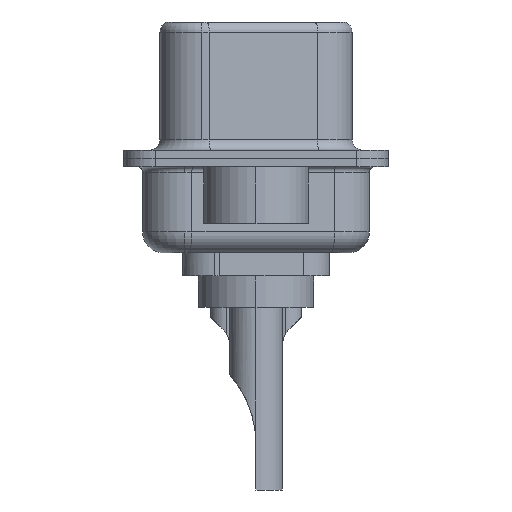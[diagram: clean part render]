
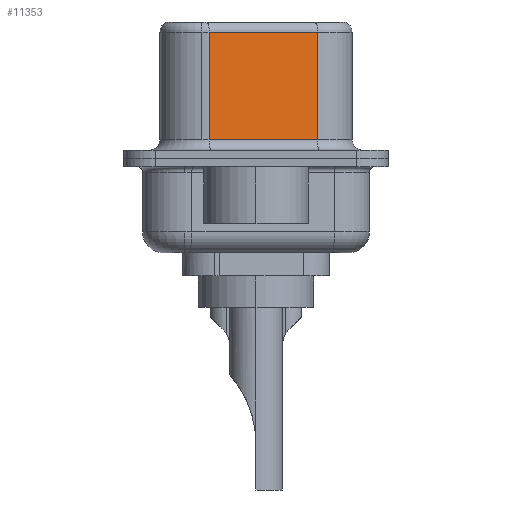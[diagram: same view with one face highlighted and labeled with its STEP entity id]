
A CAD part, left-side view. The second image highlights one B-rep face of the part: STEP entity #11353.
In plain terms, the highlighted planar face has unit normal (-0.985, -0.174, 0).
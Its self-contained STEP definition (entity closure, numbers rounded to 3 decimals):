
#414 = VERTEX_POINT ( 'NONE', #11921 ) ;
#579 = VERTEX_POINT ( 'NONE', #12509 ) ;
#940 = LINE ( 'NONE', #13242, #16454 ) ;
#2225 = ORIENTED_EDGE ( 'NONE', *, *, #14039, .T. ) ;
#2245 = CARTESIAN_POINT ( 'NONE',  ( 4.585, -2.927, 6.02 ) ) ;
#2820 = DIRECTION ( 'NONE',  ( 0., 0., -1. ) ) ;
#2828 = LINE ( 'NONE', #16336, #4476 ) ;
#3427 = EDGE_CURVE ( 'NONE', #15563, #5354, #940, .T. ) ;
#3500 = PLANE ( 'NONE',  #6195 ) ;
#3525 = CARTESIAN_POINT ( 'NONE',  ( 3.675, 2.233, 6.52 ) ) ;
#4476 = VECTOR ( 'NONE', #2820, 1000. ) ;
#4582 = EDGE_LOOP ( 'NONE', ( #11446, #7759, #16060, #2225 ) ) ;
#4767 = EDGE_CURVE ( 'NONE', #15563, #414, #2828, .T. ) ;
#5354 = VERTEX_POINT ( 'NONE', #12148 ) ;
#5702 = LINE ( 'NONE', #19414, #15691 ) ;
#6195 = AXIS2_PLACEMENT_3D ( 'NONE', #6426, #10901, #18558 ) ;
#6426 = CARTESIAN_POINT ( 'NONE',  ( 4.585, -2.927, 6.52 ) ) ;
#7759 = ORIENTED_EDGE ( 'NONE', *, *, #3427, .T. ) ;
#8699 = VECTOR ( 'NONE', #12587, 1000. ) ;
#9319 = EDGE_CURVE ( 'NONE', #5354, #579, #12764, .T. ) ;
#10901 = DIRECTION ( 'NONE',  ( 0.985, 0.174, 0. ) ) ;
#11353 = ADVANCED_FACE ( 'NONE', ( #18420 ), #3500, .F. ) ;
#11446 = ORIENTED_EDGE ( 'NONE', *, *, #4767, .F. ) ;
#11921 = CARTESIAN_POINT ( 'NONE',  ( 4.585, -2.927, 0.9 ) ) ;
#12148 = CARTESIAN_POINT ( 'NONE',  ( 3.675, 2.233, 6.02 ) ) ;
#12509 = CARTESIAN_POINT ( 'NONE',  ( 3.675, 2.233, 0.9 ) ) ;
#12587 = DIRECTION ( 'NONE',  ( 0., 0., -1. ) ) ;
#12764 = LINE ( 'NONE', #3525, #8699 ) ;
#13242 = CARTESIAN_POINT ( 'NONE',  ( 4.585, -2.927, 6.02 ) ) ;
#13343 = DIRECTION ( 'NONE',  ( 0.174, -0.985, 0. ) ) ;
#14039 = EDGE_CURVE ( 'NONE', #579, #414, #5702, .T. ) ;
#14889 = DIRECTION ( 'NONE',  ( -0.174, 0.985, 0. ) ) ;
#15563 = VERTEX_POINT ( 'NONE', #2245 ) ;
#15691 = VECTOR ( 'NONE', #13343, 1000. ) ;
#16060 = ORIENTED_EDGE ( 'NONE', *, *, #9319, .T. ) ;
#16336 = CARTESIAN_POINT ( 'NONE',  ( 4.585, -2.927, 6.52 ) ) ;
#16454 = VECTOR ( 'NONE', #14889, 1000. ) ;
#18420 = FACE_OUTER_BOUND ( 'NONE', #4582, .T. ) ;
#18558 = DIRECTION ( 'NONE',  ( -0.174, 0.985, 0. ) ) ;
#19414 = CARTESIAN_POINT ( 'NONE',  ( 4.585, -2.927, 0.9 ) ) ;
